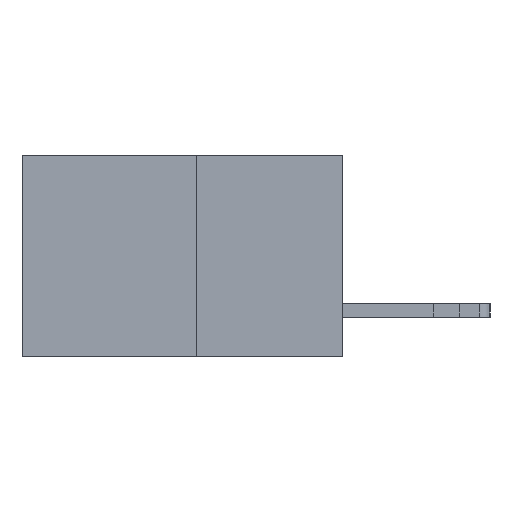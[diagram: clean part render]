
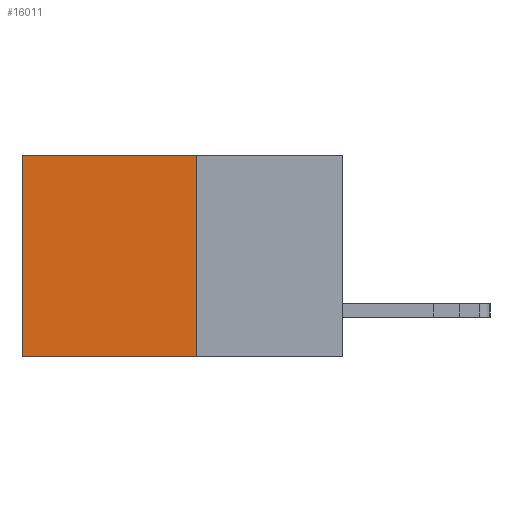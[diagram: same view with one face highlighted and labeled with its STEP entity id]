
A CAD part, left-side view. The second image highlights one B-rep face of the part: STEP entity #16011.
In plain terms, the highlighted planar face has unit normal (-1, 0, 0).
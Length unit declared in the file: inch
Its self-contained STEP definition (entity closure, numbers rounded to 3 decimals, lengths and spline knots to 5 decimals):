
#428 = CARTESIAN_POINT ( 'NONE',  ( 0.277, 0.27, -0.37 ) ) ;
#658 = ORIENTED_EDGE ( 'NONE', *, *, #24940, .F. ) ;
#1324 = DIRECTION ( 'NONE',  ( 0., 0., -1. ) ) ;
#2602 = DIRECTION ( 'NONE',  ( 0., 0., -1. ) ) ;
#2634 = CARTESIAN_POINT ( 'NONE',  ( 0.277, 0.59, 0. ) ) ;
#3551 = FACE_OUTER_BOUND ( 'NONE', #12579, .T. ) ;
#7573 = CARTESIAN_POINT ( 'NONE',  ( 0.277, 0.59, -0.37 ) ) ;
#8407 = VERTEX_POINT ( 'NONE', #24687 ) ;
#8860 = DIRECTION ( 'NONE',  ( 1., 0., 0. ) ) ;
#10669 = CARTESIAN_POINT ( 'NONE',  ( 0.277, 0.27, -0.37 ) ) ;
#11413 = EDGE_CURVE ( 'NONE', #21259, #15034, #24376, .T. ) ;
#12549 = VECTOR ( 'NONE', #1324, 39.37008 ) ;
#12579 = EDGE_LOOP ( 'NONE', ( #21096, #26001, #658, #22481 ) ) ;
#12741 = CARTESIAN_POINT ( 'NONE',  ( 0.277, 0.27, 0. ) ) ;
#12776 = DIRECTION ( 'NONE',  ( 0., 1., 0. ) ) ;
#12793 = VECTOR ( 'NONE', #2602, 39.37008 ) ;
#13006 = CARTESIAN_POINT ( 'NONE',  ( 0.277, 0.27, -0.37 ) ) ;
#15034 = VERTEX_POINT ( 'NONE', #19637 ) ;
#15927 = EDGE_CURVE ( 'NONE', #20693, #15034, #22198, .T. ) ;
#16011 = ADVANCED_FACE ( 'NONE', ( #3551 ), #21370, .F. ) ;
#16922 = DIRECTION ( 'NONE',  ( 0., 1., 0. ) ) ;
#17846 = CARTESIAN_POINT ( 'NONE',  ( 0.277, 0.27, -0.37 ) ) ;
#18338 = LINE ( 'NONE', #13006, #12793 ) ;
#19604 = LINE ( 'NONE', #12741, #26177 ) ;
#19637 = CARTESIAN_POINT ( 'NONE',  ( 0.277, 0.59, -0.37 ) ) ;
#20693 = VERTEX_POINT ( 'NONE', #17846 ) ;
#21096 = ORIENTED_EDGE ( 'NONE', *, *, #11413, .T. ) ;
#21259 = VERTEX_POINT ( 'NONE', #2634 ) ;
#21370 = PLANE ( 'NONE',  #24601 ) ;
#22198 = LINE ( 'NONE', #10669, #27136 ) ;
#22481 = ORIENTED_EDGE ( 'NONE', *, *, #23719, .T. ) ;
#23494 = DIRECTION ( 'NONE',  ( 0., 0., -1. ) ) ;
#23719 = EDGE_CURVE ( 'NONE', #8407, #21259, #19604, .T. ) ;
#24376 = LINE ( 'NONE', #7573, #12549 ) ;
#24601 = AXIS2_PLACEMENT_3D ( 'NONE', #428, #8860, #23494 ) ;
#24687 = CARTESIAN_POINT ( 'NONE',  ( 0.277, 0.27, 0. ) ) ;
#24940 = EDGE_CURVE ( 'NONE', #8407, #20693, #18338, .T. ) ;
#26001 = ORIENTED_EDGE ( 'NONE', *, *, #15927, .F. ) ;
#26177 = VECTOR ( 'NONE', #16922, 39.37008 ) ;
#27136 = VECTOR ( 'NONE', #12776, 39.37008 ) ;
